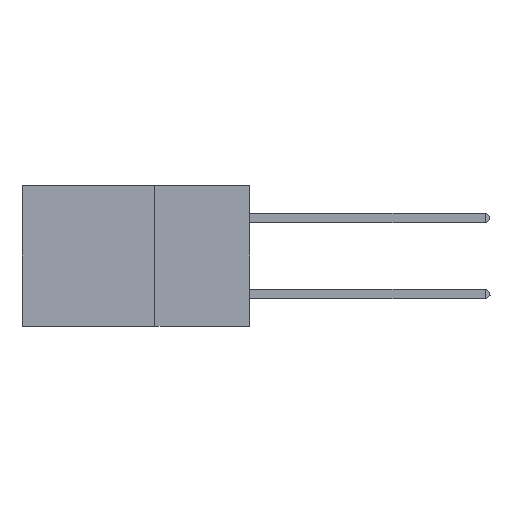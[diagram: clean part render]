
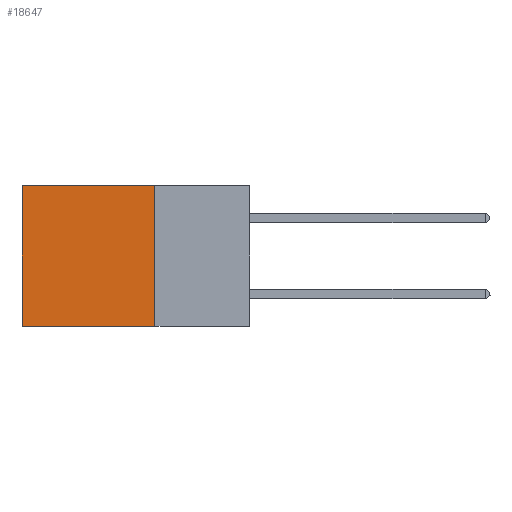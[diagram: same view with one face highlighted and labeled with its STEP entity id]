
A CAD part, left-side view. The second image highlights one B-rep face of the part: STEP entity #18647.
In plain terms, the highlighted planar face has unit normal (-1, 0, 0).
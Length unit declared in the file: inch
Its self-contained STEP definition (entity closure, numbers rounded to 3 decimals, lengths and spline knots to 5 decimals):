
#718 = VECTOR ( 'NONE', #3866, 39.37008 ) ;
#1859 = VERTEX_POINT ( 'NONE', #8211 ) ;
#2519 = LINE ( 'NONE', #6374, #29083 ) ;
#3866 = DIRECTION ( 'NONE',  ( 0., 1., 0. ) ) ;
#3934 = CARTESIAN_POINT ( 'NONE',  ( 0.2875, 0.25, 0. ) ) ;
#4155 = CARTESIAN_POINT ( 'NONE',  ( 0.2875, 0.25, -0.37 ) ) ;
#5038 = EDGE_LOOP ( 'NONE', ( #5287, #6944, #16622, #10603 ) ) ;
#5287 = ORIENTED_EDGE ( 'NONE', *, *, #21604, .T. ) ;
#5387 = LINE ( 'NONE', #4155, #718 ) ;
#6374 = CARTESIAN_POINT ( 'NONE',  ( 0.2875, 0.6, 0. ) ) ;
#6776 = EDGE_CURVE ( 'NONE', #24366, #25064, #5387, .T. ) ;
#6944 = ORIENTED_EDGE ( 'NONE', *, *, #6776, .F. ) ;
#7447 = LINE ( 'NONE', #8714, #17877 ) ;
#8211 = CARTESIAN_POINT ( 'NONE',  ( 0.2875, 0.6, 0. ) ) ;
#8714 = CARTESIAN_POINT ( 'NONE',  ( 0.2875, 0.25, 0. ) ) ;
#10603 = ORIENTED_EDGE ( 'NONE', *, *, #25149, .T. ) ;
#10917 = VERTEX_POINT ( 'NONE', #18206 ) ;
#12560 = CARTESIAN_POINT ( 'NONE',  ( 0.2875, 0.25, 0. ) ) ;
#13100 = DIRECTION ( 'NONE',  ( 0., 0., -1. ) ) ;
#13245 = DIRECTION ( 'NONE',  ( 0., 1., 0. ) ) ;
#13267 = DIRECTION ( 'NONE',  ( 0., 0., -1. ) ) ;
#14613 = CARTESIAN_POINT ( 'NONE',  ( 0.2875, 0.25, -0.37 ) ) ;
#14859 = AXIS2_PLACEMENT_3D ( 'NONE', #12560, #26612, #21988 ) ;
#15653 = FACE_OUTER_BOUND ( 'NONE', #5038, .T. ) ;
#16197 = EDGE_CURVE ( 'NONE', #10917, #24366, #26976, .T. ) ;
#16622 = ORIENTED_EDGE ( 'NONE', *, *, #16197, .F. ) ;
#17877 = VECTOR ( 'NONE', #13245, 39.37008 ) ;
#18206 = CARTESIAN_POINT ( 'NONE',  ( 0.2875, 0.25, 0. ) ) ;
#18647 = ADVANCED_FACE ( 'NONE', ( #15653 ), #26518, .F. ) ;
#19295 = CARTESIAN_POINT ( 'NONE',  ( 0.2875, 0.6, -0.37 ) ) ;
#21604 = EDGE_CURVE ( 'NONE', #1859, #25064, #2519, .T. ) ;
#21988 = DIRECTION ( 'NONE',  ( 0., 0., -1. ) ) ;
#22287 = VECTOR ( 'NONE', #13267, 39.37008 ) ;
#24366 = VERTEX_POINT ( 'NONE', #14613 ) ;
#25064 = VERTEX_POINT ( 'NONE', #19295 ) ;
#25149 = EDGE_CURVE ( 'NONE', #10917, #1859, #7447, .T. ) ;
#26518 = PLANE ( 'NONE',  #14859 ) ;
#26612 = DIRECTION ( 'NONE',  ( 1., 0., 0. ) ) ;
#26976 = LINE ( 'NONE', #3934, #22287 ) ;
#29083 = VECTOR ( 'NONE', #13100, 39.37008 ) ;
